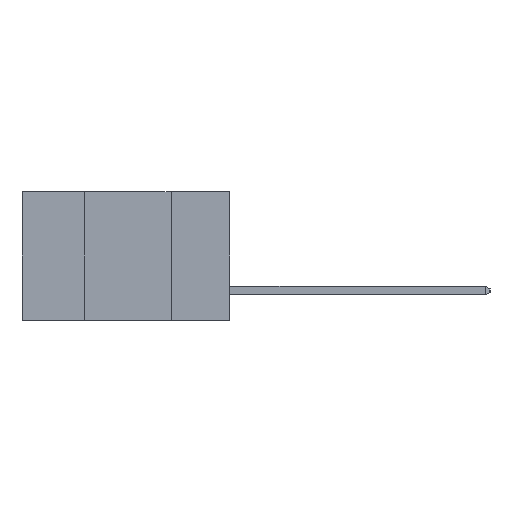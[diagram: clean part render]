
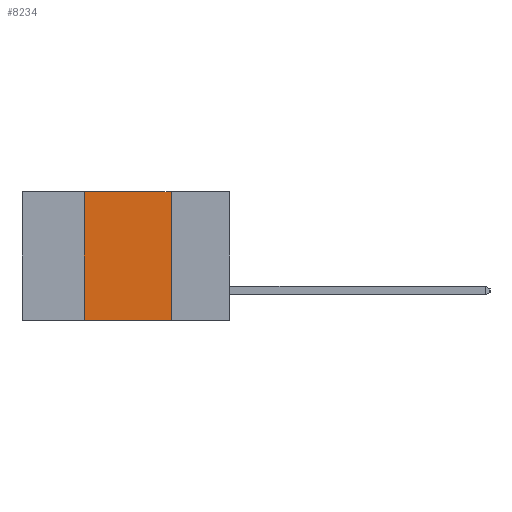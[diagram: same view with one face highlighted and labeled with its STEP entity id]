
A CAD part, left-side view. The second image highlights one B-rep face of the part: STEP entity #8234.
In plain terms, the highlighted planar face has unit normal (-1, 0, 0).
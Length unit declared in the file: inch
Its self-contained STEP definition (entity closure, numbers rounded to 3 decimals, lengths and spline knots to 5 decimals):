
#91 = EDGE_CURVE ( 'NONE', #4857, #2070, #4038, .T. ) ;
#190 = DIRECTION ( 'NONE',  ( 0., 0., 1. ) ) ;
#431 = LINE ( 'NONE', #917, #4680 ) ;
#466 = CARTESIAN_POINT ( 'NONE',  ( 0., 0.17, -0.37 ) ) ;
#837 = DIRECTION ( 'NONE',  ( 0., 0., -1. ) ) ;
#917 = CARTESIAN_POINT ( 'NONE',  ( 0., 0.17, 0. ) ) ;
#1046 = CARTESIAN_POINT ( 'NONE',  ( 0., 0.6, -0.37 ) ) ;
#1244 = AXIS2_PLACEMENT_3D ( 'NONE', #4321, #8555, #837 ) ;
#1356 = DIRECTION ( 'NONE',  ( 0., -1., 0. ) ) ;
#1379 = CARTESIAN_POINT ( 'NONE',  ( 0., 0.6, 0. ) ) ;
#1498 = CARTESIAN_POINT ( 'NONE',  ( 0., 0.42, 0. ) ) ;
#2070 = VERTEX_POINT ( 'NONE', #466 ) ;
#2975 = VERTEX_POINT ( 'NONE', #4932 ) ;
#3512 = EDGE_CURVE ( 'NONE', #5590, #2975, #9270, .T. ) ;
#3699 = ORIENTED_EDGE ( 'NONE', *, *, #91, .T. ) ;
#3720 = VECTOR ( 'NONE', #1356, 39.37008 ) ;
#4038 = LINE ( 'NONE', #1046, #7933 ) ;
#4321 = CARTESIAN_POINT ( 'NONE',  ( 0., 0.6, 0. ) ) ;
#4680 = VECTOR ( 'NONE', #8505, 39.37008 ) ;
#4857 = VERTEX_POINT ( 'NONE', #4897 ) ;
#4897 = CARTESIAN_POINT ( 'NONE',  ( 0., 0.42, -0.37 ) ) ;
#4932 = CARTESIAN_POINT ( 'NONE',  ( 0., 0.17, 0. ) ) ;
#5063 = EDGE_CURVE ( 'NONE', #4857, #5590, #6816, .T. ) ;
#5133 = PLANE ( 'NONE',  #1244 ) ;
#5590 = VERTEX_POINT ( 'NONE', #9174 ) ;
#5600 = EDGE_LOOP ( 'NONE', ( #6730, #5610, #8089, #3699 ) ) ;
#5610 = ORIENTED_EDGE ( 'NONE', *, *, #3512, .F. ) ;
#6145 = EDGE_CURVE ( 'NONE', #2975, #2070, #431, .T. ) ;
#6311 = DIRECTION ( 'NONE',  ( 0., -1., 0. ) ) ;
#6730 = ORIENTED_EDGE ( 'NONE', *, *, #6145, .F. ) ;
#6816 = LINE ( 'NONE', #1498, #8602 ) ;
#7526 = FACE_OUTER_BOUND ( 'NONE', #5600, .T. ) ;
#7933 = VECTOR ( 'NONE', #6311, 39.37008 ) ;
#8089 = ORIENTED_EDGE ( 'NONE', *, *, #5063, .F. ) ;
#8234 = ADVANCED_FACE ( 'NONE', ( #7526 ), #5133, .F. ) ;
#8505 = DIRECTION ( 'NONE',  ( 0., 0., -1. ) ) ;
#8555 = DIRECTION ( 'NONE',  ( 1., 0., 0. ) ) ;
#8602 = VECTOR ( 'NONE', #190, 39.37008 ) ;
#9174 = CARTESIAN_POINT ( 'NONE',  ( 0., 0.42, 0. ) ) ;
#9270 = LINE ( 'NONE', #1379, #3720 ) ;
